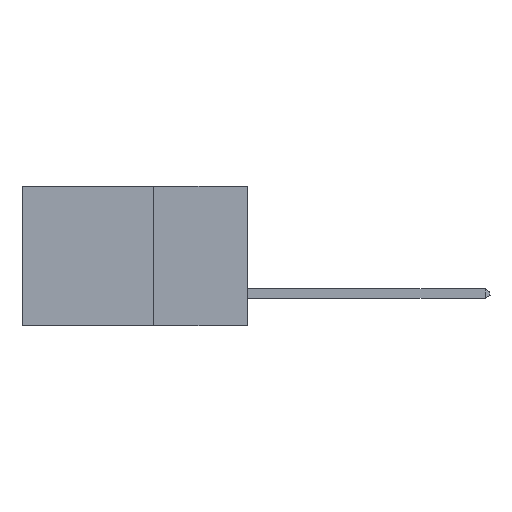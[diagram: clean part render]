
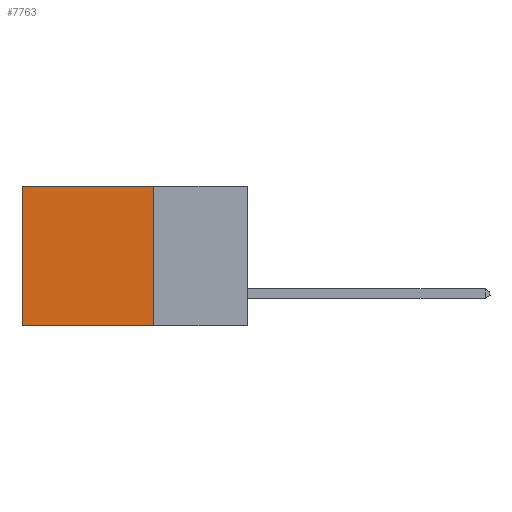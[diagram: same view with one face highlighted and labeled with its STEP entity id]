
A CAD part, left-side view. The second image highlights one B-rep face of the part: STEP entity #7763.
In plain terms, the highlighted planar face has unit normal (-1, 0, 0).
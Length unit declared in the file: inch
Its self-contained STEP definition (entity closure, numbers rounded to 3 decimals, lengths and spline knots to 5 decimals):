
#233 = ORIENTED_EDGE ( 'NONE', *, *, #10361, .T. ) ;
#704 = VERTEX_POINT ( 'NONE', #9128 ) ;
#921 = CARTESIAN_POINT ( 'NONE',  ( 0.298, 0.6, -0.37 ) ) ;
#2994 = AXIS2_PLACEMENT_3D ( 'NONE', #3304, #6833, #9195 ) ;
#3184 = EDGE_CURVE ( 'NONE', #704, #5242, #3241, .T. ) ;
#3241 = LINE ( 'NONE', #8095, #9707 ) ;
#3255 = PLANE ( 'NONE',  #2994 ) ;
#3304 = CARTESIAN_POINT ( 'NONE',  ( 0.298, 0.25, 0. ) ) ;
#3929 = EDGE_CURVE ( 'NONE', #6608, #14365, #6571, .T. ) ;
#4342 = ORIENTED_EDGE ( 'NONE', *, *, #12516, .F. ) ;
#4555 = LINE ( 'NONE', #9702, #10782 ) ;
#5242 = VERTEX_POINT ( 'NONE', #9089 ) ;
#5376 = DIRECTION ( 'NONE',  ( 0., 0., -1. ) ) ;
#6571 = LINE ( 'NONE', #13749, #13106 ) ;
#6608 = VERTEX_POINT ( 'NONE', #13234 ) ;
#6833 = DIRECTION ( 'NONE',  ( 1., 0., 0. ) ) ;
#7763 = ADVANCED_FACE ( 'NONE', ( #13046 ), #3255, .F. ) ;
#8095 = CARTESIAN_POINT ( 'NONE',  ( 0.298, 0.25, 0. ) ) ;
#8491 = ORIENTED_EDGE ( 'NONE', *, *, #3184, .F. ) ;
#9089 = CARTESIAN_POINT ( 'NONE',  ( 0.298, 0.25, -0.37 ) ) ;
#9092 = ORIENTED_EDGE ( 'NONE', *, *, #3929, .T. ) ;
#9128 = CARTESIAN_POINT ( 'NONE',  ( 0.298, 0.25, 0. ) ) ;
#9139 = DIRECTION ( 'NONE',  ( 0., 0., -1. ) ) ;
#9195 = DIRECTION ( 'NONE',  ( 0., 0., -1. ) ) ;
#9690 = CARTESIAN_POINT ( 'NONE',  ( 0.298, 0.25, -0.37 ) ) ;
#9702 = CARTESIAN_POINT ( 'NONE',  ( 0.298, 0.25, 0. ) ) ;
#9707 = VECTOR ( 'NONE', #5376, 39.37008 ) ;
#10361 = EDGE_CURVE ( 'NONE', #704, #6608, #4555, .T. ) ;
#10782 = VECTOR ( 'NONE', #13031, 39.37008 ) ;
#11673 = EDGE_LOOP ( 'NONE', ( #9092, #4342, #8491, #233 ) ) ;
#11960 = DIRECTION ( 'NONE',  ( 0., 1., 0. ) ) ;
#12516 = EDGE_CURVE ( 'NONE', #5242, #14365, #14387, .T. ) ;
#13031 = DIRECTION ( 'NONE',  ( 0., 1., 0. ) ) ;
#13046 = FACE_OUTER_BOUND ( 'NONE', #11673, .T. ) ;
#13106 = VECTOR ( 'NONE', #9139, 39.37008 ) ;
#13234 = CARTESIAN_POINT ( 'NONE',  ( 0.298, 0.6, 0. ) ) ;
#13749 = CARTESIAN_POINT ( 'NONE',  ( 0.298, 0.6, 0. ) ) ;
#13849 = VECTOR ( 'NONE', #11960, 39.37008 ) ;
#14365 = VERTEX_POINT ( 'NONE', #921 ) ;
#14387 = LINE ( 'NONE', #9690, #13849 ) ;
